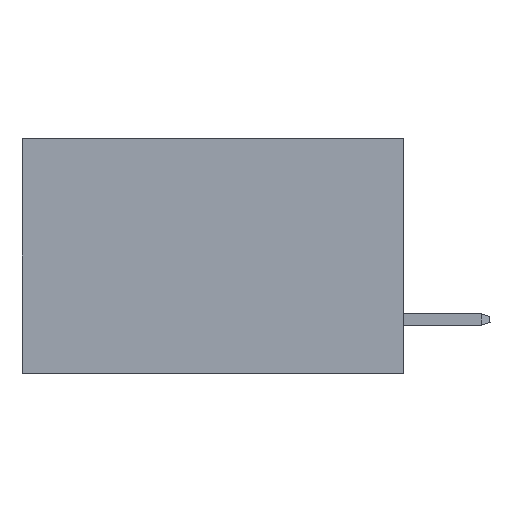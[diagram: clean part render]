
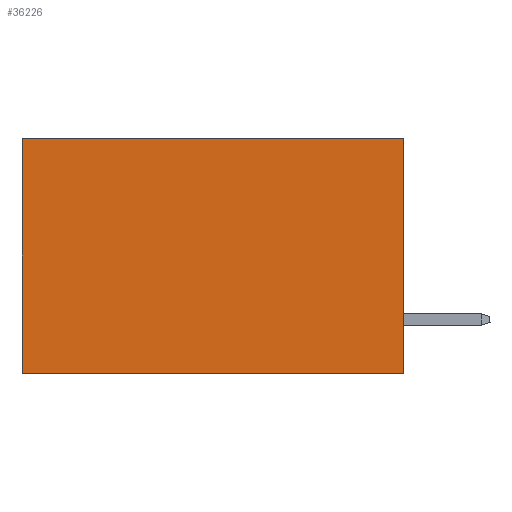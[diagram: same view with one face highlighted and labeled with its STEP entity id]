
A CAD part, left-side view. The second image highlights one B-rep face of the part: STEP entity #36226.
In plain terms, the highlighted planar face has unit normal (-1, 0, 0).
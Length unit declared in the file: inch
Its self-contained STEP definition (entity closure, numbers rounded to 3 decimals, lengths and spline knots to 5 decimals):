
#326 = ORIENTED_EDGE ( 'NONE', *, *, #38121, .T. ) ;
#1294 = VECTOR ( 'NONE', #44975, 39.37008 ) ;
#1615 = CARTESIAN_POINT ( 'NONE',  ( 0.2875, 0., 0. ) ) ;
#1866 = CARTESIAN_POINT ( 'NONE',  ( 0.2875, 0., -0.37 ) ) ;
#2284 = ORIENTED_EDGE ( 'NONE', *, *, #29363, .F. ) ;
#3209 = DIRECTION ( 'NONE',  ( 1., 0., 0. ) ) ;
#3347 = VECTOR ( 'NONE', #22579, 39.37008 ) ;
#3653 = DIRECTION ( 'NONE',  ( 0., 0., -1. ) ) ;
#3868 = CARTESIAN_POINT ( 'NONE',  ( 0.2875, 0., 0. ) ) ;
#6846 = PLANE ( 'NONE',  #12730 ) ;
#8239 = LINE ( 'NONE', #8696, #3347 ) ;
#8696 = CARTESIAN_POINT ( 'NONE',  ( 0.2875, 0.6, 0. ) ) ;
#10779 = EDGE_CURVE ( 'NONE', #40715, #28385, #28101, .T. ) ;
#12662 = LINE ( 'NONE', #13113, #13873 ) ;
#12730 = AXIS2_PLACEMENT_3D ( 'NONE', #3868, #3209, #3653 ) ;
#13113 = CARTESIAN_POINT ( 'NONE',  ( 0.2875, 0., -0.37 ) ) ;
#13283 = EDGE_LOOP ( 'NONE', ( #25287, #2284, #43876, #326 ) ) ;
#13873 = VECTOR ( 'NONE', #29979, 39.37008 ) ;
#18880 = CARTESIAN_POINT ( 'NONE',  ( 0.2875, 0.6, -0.37 ) ) ;
#21587 = VECTOR ( 'NONE', #22553, 39.37008 ) ;
#22553 = DIRECTION ( 'NONE',  ( 0., 1., 0. ) ) ;
#22579 = DIRECTION ( 'NONE',  ( 0., 0., -1. ) ) ;
#23836 = EDGE_CURVE ( 'NONE', #25157, #43670, #8239, .T. ) ;
#25157 = VERTEX_POINT ( 'NONE', #43389 ) ;
#25287 = ORIENTED_EDGE ( 'NONE', *, *, #23836, .T. ) ;
#28101 = LINE ( 'NONE', #31086, #1294 ) ;
#28385 = VERTEX_POINT ( 'NONE', #1866 ) ;
#29363 = EDGE_CURVE ( 'NONE', #28385, #43670, #12662, .T. ) ;
#29979 = DIRECTION ( 'NONE',  ( 0., 1., 0. ) ) ;
#31086 = CARTESIAN_POINT ( 'NONE',  ( 0.2875, 0., 0. ) ) ;
#32590 = LINE ( 'NONE', #1615, #21587 ) ;
#34407 = FACE_OUTER_BOUND ( 'NONE', #13283, .T. ) ;
#36226 = ADVANCED_FACE ( 'NONE', ( #34407 ), #6846, .F. ) ;
#38121 = EDGE_CURVE ( 'NONE', #40715, #25157, #32590, .T. ) ;
#40715 = VERTEX_POINT ( 'NONE', #43463 ) ;
#43389 = CARTESIAN_POINT ( 'NONE',  ( 0.2875, 0.6, 0. ) ) ;
#43463 = CARTESIAN_POINT ( 'NONE',  ( 0.2875, 0., 0. ) ) ;
#43670 = VERTEX_POINT ( 'NONE', #18880 ) ;
#43876 = ORIENTED_EDGE ( 'NONE', *, *, #10779, .F. ) ;
#44975 = DIRECTION ( 'NONE',  ( 0., 0., -1. ) ) ;
